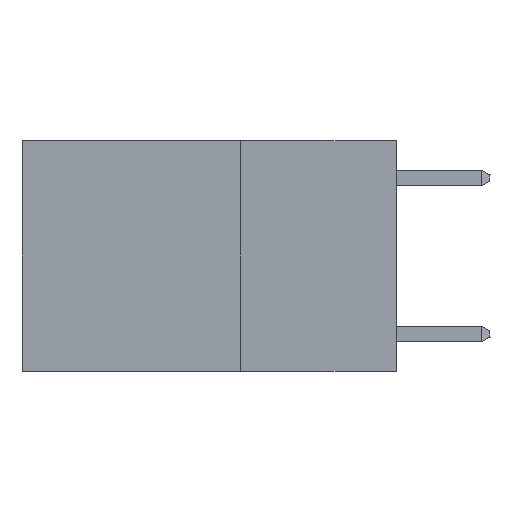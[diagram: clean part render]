
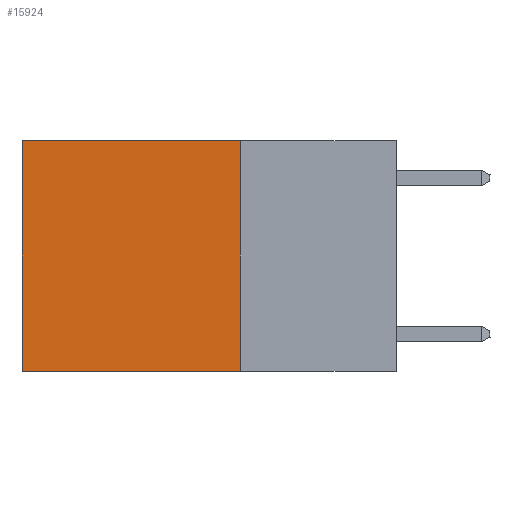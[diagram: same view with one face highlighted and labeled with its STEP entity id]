
A CAD part, left-side view. The second image highlights one B-rep face of the part: STEP entity #15924.
In plain terms, the highlighted planar face has unit normal (-1, 0, 0).
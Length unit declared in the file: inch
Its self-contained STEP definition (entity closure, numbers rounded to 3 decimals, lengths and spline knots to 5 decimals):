
#1060 = CARTESIAN_POINT ( 'NONE',  ( 0.2625, 0.25, 0. ) ) ;
#1066 = VECTOR ( 'NONE', #12652, 39.37008 ) ;
#2210 = EDGE_CURVE ( 'NONE', #3490, #9960, #14499, .T. ) ;
#2329 = ORIENTED_EDGE ( 'NONE', *, *, #2210, .T. ) ;
#2557 = LINE ( 'NONE', #14978, #9190 ) ;
#3342 = EDGE_LOOP ( 'NONE', ( #20096, #6179, #5069, #2329 ) ) ;
#3490 = VERTEX_POINT ( 'NONE', #12017 ) ;
#4133 = DIRECTION ( 'NONE',  ( 1., 0., 0. ) ) ;
#4155 = VECTOR ( 'NONE', #11532, 39.37008 ) ;
#5069 = ORIENTED_EDGE ( 'NONE', *, *, #6455, .F. ) ;
#6179 = ORIENTED_EDGE ( 'NONE', *, *, #11459, .F. ) ;
#6455 = EDGE_CURVE ( 'NONE', #3490, #15704, #8752, .T. ) ;
#6713 = CARTESIAN_POINT ( 'NONE',  ( 0.2625, 0.25, -0.37 ) ) ;
#7133 = PLANE ( 'NONE',  #15427 ) ;
#7960 = EDGE_CURVE ( 'NONE', #9960, #11952, #2557, .T. ) ;
#8748 = DIRECTION ( 'NONE',  ( 0., 0., -1. ) ) ;
#8752 = LINE ( 'NONE', #1060, #15601 ) ;
#8842 = CARTESIAN_POINT ( 'NONE',  ( 0.2625, 0.6, -0.37 ) ) ;
#9190 = VECTOR ( 'NONE', #8748, 39.37008 ) ;
#9628 = CARTESIAN_POINT ( 'NONE',  ( 0.2625, 0.25, -0.37 ) ) ;
#9960 = VERTEX_POINT ( 'NONE', #14227 ) ;
#10334 = DIRECTION ( 'NONE',  ( 0., 0., -1. ) ) ;
#11459 = EDGE_CURVE ( 'NONE', #15704, #11952, #13135, .T. ) ;
#11532 = DIRECTION ( 'NONE',  ( 0., 1., 0. ) ) ;
#11952 = VERTEX_POINT ( 'NONE', #8842 ) ;
#12017 = CARTESIAN_POINT ( 'NONE',  ( 0.2625, 0.25, 0. ) ) ;
#12652 = DIRECTION ( 'NONE',  ( 0., 1., 0. ) ) ;
#12951 = CARTESIAN_POINT ( 'NONE',  ( 0.2625, 0.25, 0. ) ) ;
#13135 = LINE ( 'NONE', #6713, #4155 ) ;
#14227 = CARTESIAN_POINT ( 'NONE',  ( 0.2625, 0.6, 0. ) ) ;
#14499 = LINE ( 'NONE', #12951, #1066 ) ;
#14978 = CARTESIAN_POINT ( 'NONE',  ( 0.2625, 0.6, 0. ) ) ;
#15427 = AXIS2_PLACEMENT_3D ( 'NONE', #19625, #4133, #10334 ) ;
#15601 = VECTOR ( 'NONE', #18068, 39.37008 ) ;
#15704 = VERTEX_POINT ( 'NONE', #9628 ) ;
#15924 = ADVANCED_FACE ( 'NONE', ( #18099 ), #7133, .F. ) ;
#18068 = DIRECTION ( 'NONE',  ( 0., 0., -1. ) ) ;
#18099 = FACE_OUTER_BOUND ( 'NONE', #3342, .T. ) ;
#19625 = CARTESIAN_POINT ( 'NONE',  ( 0.2625, 0.25, 0. ) ) ;
#20096 = ORIENTED_EDGE ( 'NONE', *, *, #7960, .T. ) ;
